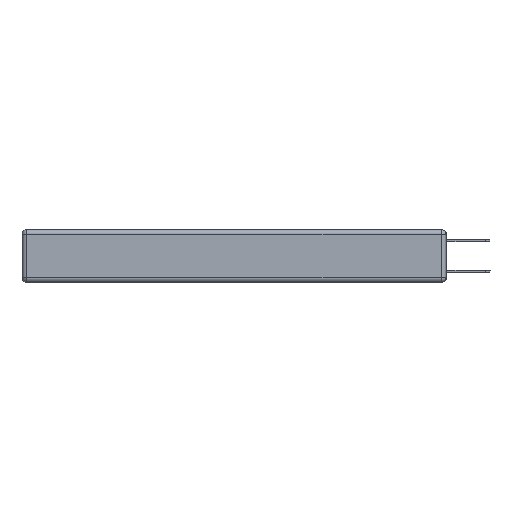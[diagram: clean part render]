
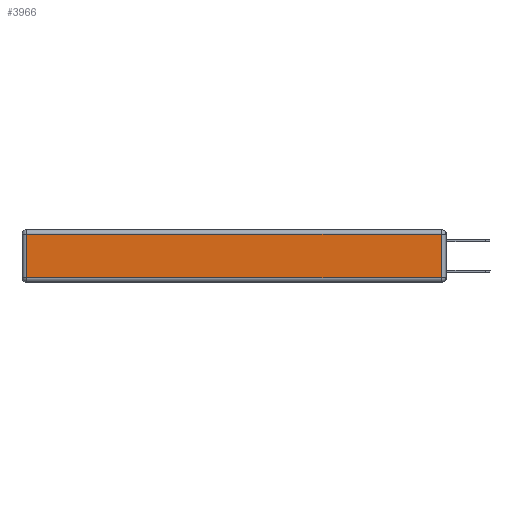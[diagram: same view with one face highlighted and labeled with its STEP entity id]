
A CAD part, left-side view. The second image highlights one B-rep face of the part: STEP entity #3966.
In plain terms, the highlighted planar face has unit normal (-1, 0, 0).
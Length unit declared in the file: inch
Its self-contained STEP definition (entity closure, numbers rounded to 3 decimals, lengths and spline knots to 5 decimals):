
#79 = EDGE_CURVE ( 'NONE', #4137, #13475, #7626, .T. ) ;
#951 = ORIENTED_EDGE ( 'NONE', *, *, #79, .T. ) ;
#1020 = CARTESIAN_POINT ( 'NONE',  ( 0., 0., -0.343 ) ) ;
#1336 = CARTESIAN_POINT ( 'NONE',  ( 0., 2.72, -0.343 ) ) ;
#1833 = DIRECTION ( 'NONE',  ( 0., 0., 1. ) ) ;
#2341 = CARTESIAN_POINT ( 'NONE',  ( 0., 0., -0.313 ) ) ;
#3298 = PLANE ( 'NONE',  #11486 ) ;
#3966 = ADVANCED_FACE ( 'NONE', ( #5371 ), #3298, .T. ) ;
#4100 = ORIENTED_EDGE ( 'NONE', *, *, #5272, .T. ) ;
#4137 = VERTEX_POINT ( 'NONE', #11396 ) ;
#4743 = VECTOR ( 'NONE', #7764, 39.37008 ) ;
#4793 = ORIENTED_EDGE ( 'NONE', *, *, #5515, .T. ) ;
#4974 = CARTESIAN_POINT ( 'NONE',  ( 0., 2.75, -0.03 ) ) ;
#4975 = VECTOR ( 'NONE', #8342, 39.37008 ) ;
#5272 = EDGE_CURVE ( 'NONE', #9191, #4137, #12261, .T. ) ;
#5371 = FACE_OUTER_BOUND ( 'NONE', #7425, .T. ) ;
#5515 = EDGE_CURVE ( 'NONE', #9148, #9191, #7860, .T. ) ;
#5553 = DIRECTION ( 'NONE',  ( -1., 0., 0. ) ) ;
#6196 = ORIENTED_EDGE ( 'NONE', *, *, #13345, .T. ) ;
#6472 = DIRECTION ( 'NONE',  ( 0., 0., 1. ) ) ;
#7140 = CARTESIAN_POINT ( 'NONE',  ( 0., 0.03, -0.343 ) ) ;
#7365 = CARTESIAN_POINT ( 'NONE',  ( 0., 0.03, -0.03 ) ) ;
#7425 = EDGE_LOOP ( 'NONE', ( #951, #6196, #4793, #4100 ) ) ;
#7626 = LINE ( 'NONE', #2341, #4743 ) ;
#7764 = DIRECTION ( 'NONE',  ( 0., -1., 0. ) ) ;
#7860 = LINE ( 'NONE', #4974, #4975 ) ;
#8342 = DIRECTION ( 'NONE',  ( 0., 1., 0. ) ) ;
#9148 = VERTEX_POINT ( 'NONE', #7365 ) ;
#9191 = VERTEX_POINT ( 'NONE', #9519 ) ;
#9519 = CARTESIAN_POINT ( 'NONE',  ( 0., 2.72, -0.03 ) ) ;
#10160 = LINE ( 'NONE', #7140, #12030 ) ;
#11078 = VECTOR ( 'NONE', #11092, 39.37008 ) ;
#11092 = DIRECTION ( 'NONE',  ( 0., 0., -1. ) ) ;
#11396 = CARTESIAN_POINT ( 'NONE',  ( 0., 2.72, -0.313 ) ) ;
#11486 = AXIS2_PLACEMENT_3D ( 'NONE', #1020, #5553, #6472 ) ;
#12030 = VECTOR ( 'NONE', #1833, 39.37008 ) ;
#12261 = LINE ( 'NONE', #1336, #11078 ) ;
#12971 = CARTESIAN_POINT ( 'NONE',  ( 0., 0.03, -0.313 ) ) ;
#13345 = EDGE_CURVE ( 'NONE', #13475, #9148, #10160, .T. ) ;
#13475 = VERTEX_POINT ( 'NONE', #12971 ) ;
